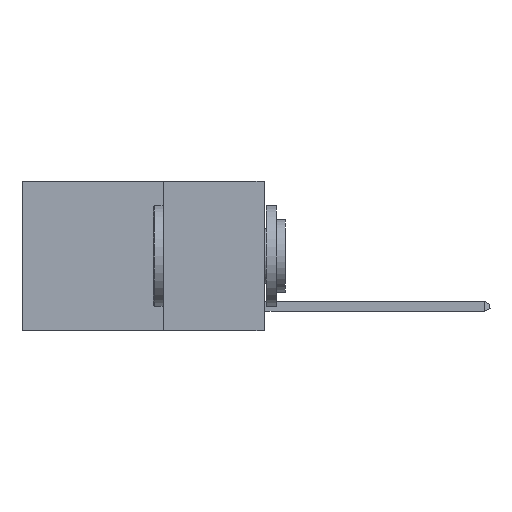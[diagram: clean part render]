
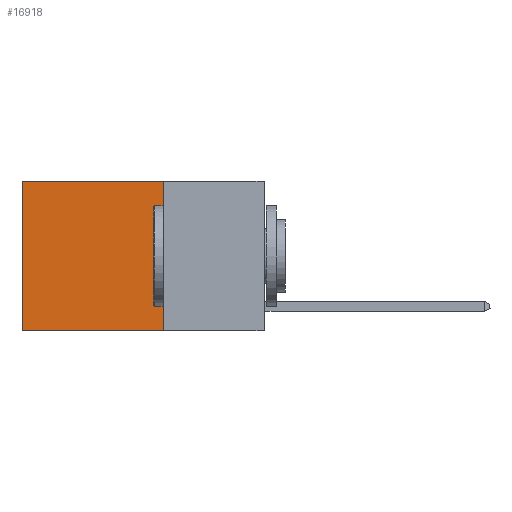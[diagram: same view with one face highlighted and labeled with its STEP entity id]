
A CAD part, left-side view. The second image highlights one B-rep face of the part: STEP entity #16918.
In plain terms, the highlighted planar face has unit normal (-1, 0, 0).
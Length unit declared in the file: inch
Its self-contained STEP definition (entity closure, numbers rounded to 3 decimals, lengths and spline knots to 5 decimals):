
#933 = LINE ( 'NONE', #19085, #12806 ) ;
#2911 = DIRECTION ( 'NONE',  ( 0., 0., -1. ) ) ;
#3315 = EDGE_CURVE ( 'NONE', #22841, #24049, #23059, .T. ) ;
#3580 = DIRECTION ( 'NONE',  ( 0., 1., 0. ) ) ;
#4014 = DIRECTION ( 'NONE',  ( 1., 0., 0. ) ) ;
#5539 = LINE ( 'NONE', #26492, #18190 ) ;
#6279 = CARTESIAN_POINT ( 'NONE',  ( 0.2625, 0.6, 0. ) ) ;
#7507 = AXIS2_PLACEMENT_3D ( 'NONE', #18269, #4014, #20626 ) ;
#8663 = LINE ( 'NONE', #16982, #20554 ) ;
#9293 = ORIENTED_EDGE ( 'NONE', *, *, #3315, .F. ) ;
#11104 = VERTEX_POINT ( 'NONE', #18565 ) ;
#12806 = VECTOR ( 'NONE', #21436, 39.37008 ) ;
#15829 = EDGE_CURVE ( 'NONE', #11104, #29837, #8663, .T. ) ;
#16918 = ADVANCED_FACE ( 'NONE', ( #22331 ), #22803, .F. ) ;
#16982 = CARTESIAN_POINT ( 'NONE',  ( 0.2625, 0.25, 0. ) ) ;
#18121 = EDGE_CURVE ( 'NONE', #29837, #24049, #5539, .T. ) ;
#18190 = VECTOR ( 'NONE', #2911, 39.37008 ) ;
#18269 = CARTESIAN_POINT ( 'NONE',  ( 0.2625, 0.25, 0. ) ) ;
#18565 = CARTESIAN_POINT ( 'NONE',  ( 0.2625, 0.25, 0. ) ) ;
#19020 = ORIENTED_EDGE ( 'NONE', *, *, #15829, .T. ) ;
#19085 = CARTESIAN_POINT ( 'NONE',  ( 0.2625, 0.25, 0. ) ) ;
#20554 = VECTOR ( 'NONE', #28690, 39.37008 ) ;
#20626 = DIRECTION ( 'NONE',  ( 0., 0., -1. ) ) ;
#21436 = DIRECTION ( 'NONE',  ( 0., 0., -1. ) ) ;
#22322 = VECTOR ( 'NONE', #3580, 39.37008 ) ;
#22331 = FACE_OUTER_BOUND ( 'NONE', #26081, .T. ) ;
#22555 = CARTESIAN_POINT ( 'NONE',  ( 0.2625, 0.25, -0.37 ) ) ;
#22803 = PLANE ( 'NONE',  #7507 ) ;
#22841 = VERTEX_POINT ( 'NONE', #28727 ) ;
#23059 = LINE ( 'NONE', #22555, #22322 ) ;
#23632 = ORIENTED_EDGE ( 'NONE', *, *, #24322, .F. ) ;
#23994 = ORIENTED_EDGE ( 'NONE', *, *, #18121, .T. ) ;
#24049 = VERTEX_POINT ( 'NONE', #29841 ) ;
#24322 = EDGE_CURVE ( 'NONE', #11104, #22841, #933, .T. ) ;
#26081 = EDGE_LOOP ( 'NONE', ( #23994, #9293, #23632, #19020 ) ) ;
#26492 = CARTESIAN_POINT ( 'NONE',  ( 0.2625, 0.6, 0. ) ) ;
#28690 = DIRECTION ( 'NONE',  ( 0., 1., 0. ) ) ;
#28727 = CARTESIAN_POINT ( 'NONE',  ( 0.2625, 0.25, -0.37 ) ) ;
#29837 = VERTEX_POINT ( 'NONE', #6279 ) ;
#29841 = CARTESIAN_POINT ( 'NONE',  ( 0.2625, 0.6, -0.37 ) ) ;
